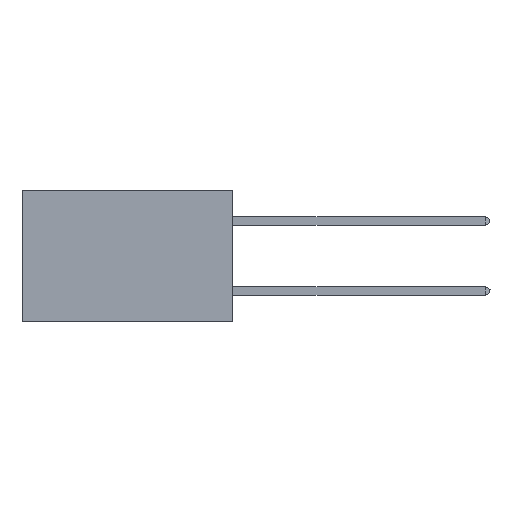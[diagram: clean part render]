
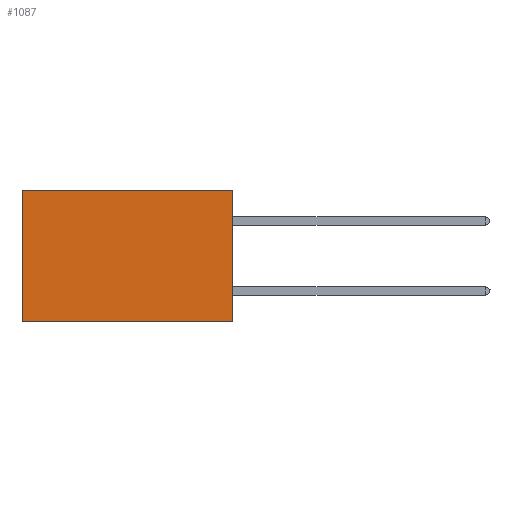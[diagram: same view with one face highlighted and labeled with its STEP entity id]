
A CAD part, left-side view. The second image highlights one B-rep face of the part: STEP entity #1087.
In plain terms, the highlighted planar face has unit normal (-1, 0, 0).
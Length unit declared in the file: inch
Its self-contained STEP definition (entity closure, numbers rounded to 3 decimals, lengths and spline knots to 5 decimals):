
#336 = LINE ( 'NONE', #16048, #5948 ) ;
#672 = DIRECTION ( 'NONE',  ( 0., 1., 0. ) ) ;
#1087 = ADVANCED_FACE ( 'NONE', ( #3678 ), #6518, .F. ) ;
#2020 = LINE ( 'NONE', #10516, #9604 ) ;
#2944 = VERTEX_POINT ( 'NONE', #10111 ) ;
#3678 = FACE_OUTER_BOUND ( 'NONE', #18076, .T. ) ;
#3716 = VECTOR ( 'NONE', #672, 39.37008 ) ;
#5948 = VECTOR ( 'NONE', #11429, 39.37008 ) ;
#5958 = LINE ( 'NONE', #8242, #3716 ) ;
#6518 = PLANE ( 'NONE',  #6555 ) ;
#6555 = AXIS2_PLACEMENT_3D ( 'NONE', #10618, #9137, #13527 ) ;
#7508 = ORIENTED_EDGE ( 'NONE', *, *, #12288, .F. ) ;
#8242 = CARTESIAN_POINT ( 'NONE',  ( 0.2875, 0., 0. ) ) ;
#8363 = LINE ( 'NONE', #16817, #13915 ) ;
#8692 = ORIENTED_EDGE ( 'NONE', *, *, #8908, .T. ) ;
#8779 = CARTESIAN_POINT ( 'NONE',  ( 0.2875, 0., 0. ) ) ;
#8908 = EDGE_CURVE ( 'NONE', #14028, #2944, #5958, .T. ) ;
#9137 = DIRECTION ( 'NONE',  ( 1., 0., 0. ) ) ;
#9604 = VECTOR ( 'NONE', #11815, 39.37008 ) ;
#10111 = CARTESIAN_POINT ( 'NONE',  ( 0.2875, 0.6, 0. ) ) ;
#10516 = CARTESIAN_POINT ( 'NONE',  ( 0.2875, 0.6, -0.375 ) ) ;
#10618 = CARTESIAN_POINT ( 'NONE',  ( 0.2875, 0., -0.375 ) ) ;
#10698 = VERTEX_POINT ( 'NONE', #13797 ) ;
#11429 = DIRECTION ( 'NONE',  ( 0., 0., -1. ) ) ;
#11815 = DIRECTION ( 'NONE',  ( 0., 0., -1. ) ) ;
#11991 = CARTESIAN_POINT ( 'NONE',  ( 0.2875, 0., -0.375 ) ) ;
#12288 = EDGE_CURVE ( 'NONE', #15403, #10698, #8363, .T. ) ;
#13483 = EDGE_CURVE ( 'NONE', #2944, #10698, #2020, .T. ) ;
#13527 = DIRECTION ( 'NONE',  ( 0., 0., -1. ) ) ;
#13773 = DIRECTION ( 'NONE',  ( 0., 1., 0. ) ) ;
#13797 = CARTESIAN_POINT ( 'NONE',  ( 0.2875, 0.6, -0.375 ) ) ;
#13915 = VECTOR ( 'NONE', #13773, 39.37008 ) ;
#14028 = VERTEX_POINT ( 'NONE', #8779 ) ;
#14714 = ORIENTED_EDGE ( 'NONE', *, *, #13483, .T. ) ;
#15403 = VERTEX_POINT ( 'NONE', #11991 ) ;
#15776 = EDGE_CURVE ( 'NONE', #14028, #15403, #336, .T. ) ;
#16048 = CARTESIAN_POINT ( 'NONE',  ( 0.2875, 0., -0.375 ) ) ;
#16817 = CARTESIAN_POINT ( 'NONE',  ( 0.2875, 0., -0.375 ) ) ;
#17463 = ORIENTED_EDGE ( 'NONE', *, *, #15776, .F. ) ;
#18076 = EDGE_LOOP ( 'NONE', ( #14714, #7508, #17463, #8692 ) ) ;
